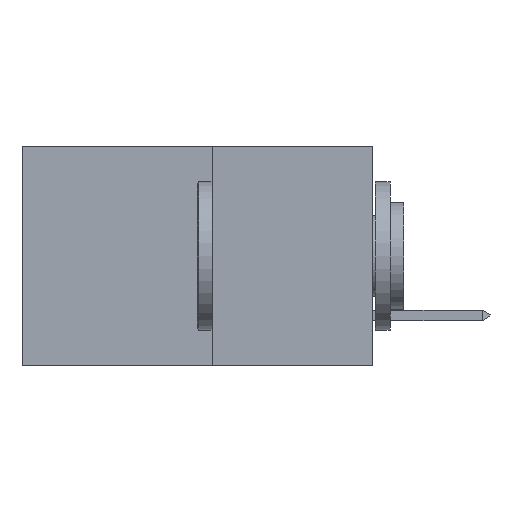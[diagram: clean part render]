
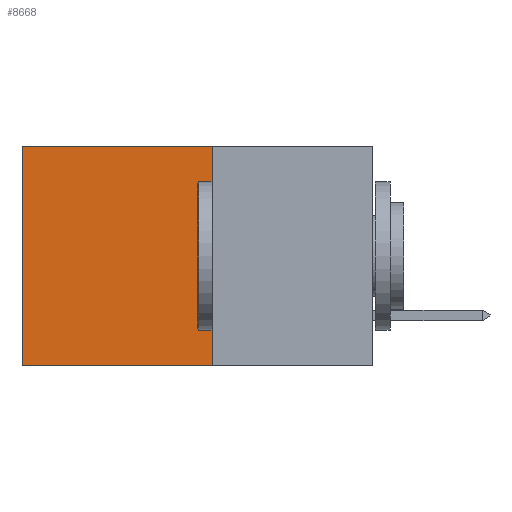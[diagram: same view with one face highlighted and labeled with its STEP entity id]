
A CAD part, left-side view. The second image highlights one B-rep face of the part: STEP entity #8668.
In plain terms, the highlighted planar face has unit normal (-1, 0, 0).
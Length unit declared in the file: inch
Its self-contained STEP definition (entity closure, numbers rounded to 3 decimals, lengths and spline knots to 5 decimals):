
#198 = LINE ( 'NONE', #24725, #16402 ) ;
#281 = EDGE_CURVE ( 'NONE', #25642, #1814, #17228, .T. ) ;
#771 = DIRECTION ( 'NONE',  ( 0., 1., 0. ) ) ;
#1015 = ORIENTED_EDGE ( 'NONE', *, *, #4753, .T. ) ;
#1814 = VERTEX_POINT ( 'NONE', #20922 ) ;
#2598 = ORIENTED_EDGE ( 'NONE', *, *, #281, .F. ) ;
#4753 = EDGE_CURVE ( 'NONE', #19722, #1814, #18104, .T. ) ;
#4999 = CARTESIAN_POINT ( 'NONE',  ( 0.277, 0.27, 0. ) ) ;
#6030 = AXIS2_PLACEMENT_3D ( 'NONE', #6276, #6057, #6031 ) ;
#6031 = DIRECTION ( 'NONE',  ( 0., 0., -1. ) ) ;
#6057 = DIRECTION ( 'NONE',  ( 1., 0., 0. ) ) ;
#6124 = CARTESIAN_POINT ( 'NONE',  ( 0.277, 0.27, -0.37 ) ) ;
#6159 = PLANE ( 'NONE',  #6030 ) ;
#6276 = CARTESIAN_POINT ( 'NONE',  ( 0.277, 0.27, -0.37 ) ) ;
#6888 = CARTESIAN_POINT ( 'NONE',  ( 0.277, 0.27, -0.37 ) ) ;
#7096 = CARTESIAN_POINT ( 'NONE',  ( 0.277, 0.27, 0. ) ) ;
#8668 = ADVANCED_FACE ( 'NONE', ( #21817 ), #6159, .F. ) ;
#10225 = EDGE_CURVE ( 'NONE', #12693, #25642, #198, .T. ) ;
#11615 = VECTOR ( 'NONE', #18247, 39.37008 ) ;
#12547 = VECTOR ( 'NONE', #25242, 39.37008 ) ;
#12693 = VERTEX_POINT ( 'NONE', #4999 ) ;
#14029 = EDGE_LOOP ( 'NONE', ( #1015, #2598, #18510, #15589 ) ) ;
#15337 = VECTOR ( 'NONE', #771, 39.37008 ) ;
#15589 = ORIENTED_EDGE ( 'NONE', *, *, #23171, .T. ) ;
#15710 = CARTESIAN_POINT ( 'NONE',  ( 0.277, 0.59, 0. ) ) ;
#16402 = VECTOR ( 'NONE', #20592, 39.37008 ) ;
#17228 = LINE ( 'NONE', #6888, #11615 ) ;
#18104 = LINE ( 'NONE', #25475, #12547 ) ;
#18247 = DIRECTION ( 'NONE',  ( 0., 1., 0. ) ) ;
#18510 = ORIENTED_EDGE ( 'NONE', *, *, #10225, .F. ) ;
#19722 = VERTEX_POINT ( 'NONE', #15710 ) ;
#20592 = DIRECTION ( 'NONE',  ( 0., 0., -1. ) ) ;
#20922 = CARTESIAN_POINT ( 'NONE',  ( 0.277, 0.59, -0.37 ) ) ;
#21817 = FACE_OUTER_BOUND ( 'NONE', #14029, .T. ) ;
#23171 = EDGE_CURVE ( 'NONE', #12693, #19722, #26472, .T. ) ;
#24725 = CARTESIAN_POINT ( 'NONE',  ( 0.277, 0.27, -0.37 ) ) ;
#25242 = DIRECTION ( 'NONE',  ( 0., 0., -1. ) ) ;
#25475 = CARTESIAN_POINT ( 'NONE',  ( 0.277, 0.59, -0.37 ) ) ;
#25642 = VERTEX_POINT ( 'NONE', #6124 ) ;
#26472 = LINE ( 'NONE', #7096, #15337 ) ;
